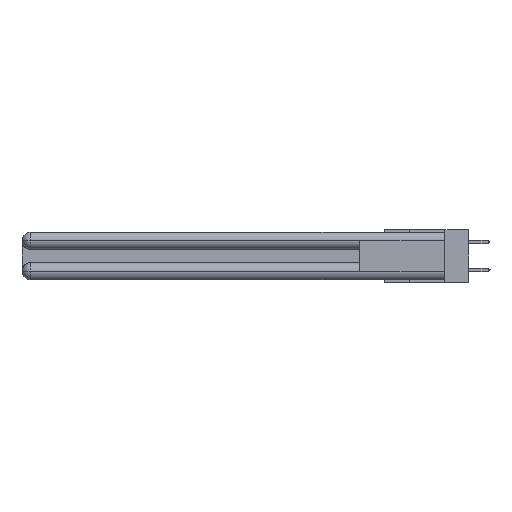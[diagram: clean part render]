
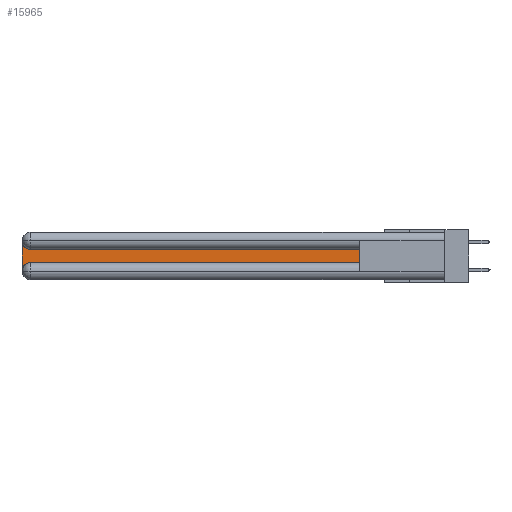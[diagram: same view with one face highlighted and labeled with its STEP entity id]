
A CAD part, left-side view. The second image highlights one B-rep face of the part: STEP entity #15965.
In plain terms, the highlighted planar face has unit normal (-1, 0, 0).
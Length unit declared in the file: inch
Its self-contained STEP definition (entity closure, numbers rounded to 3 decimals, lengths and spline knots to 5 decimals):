
#77 = CARTESIAN_POINT ( 'NONE',  ( 0.075, 2.94, -0.2775 ) ) ;
#426 = DIRECTION ( 'NONE',  ( 0., 1., 0. ) ) ;
#464 = VECTOR ( 'NONE', #27514, 39.37008 ) ;
#1423 = VERTEX_POINT ( 'NONE', #12415 ) ;
#1470 = CARTESIAN_POINT ( 'NONE',  ( 0.075, 2.94, -0.0625 ) ) ;
#2948 = DIRECTION ( 'NONE',  ( 1., 0., 0. ) ) ;
#3179 = VERTEX_POINT ( 'NONE', #11941 ) ;
#4895 = EDGE_CURVE ( 'NONE', #31831, #22219, #6930, .T. ) ;
#5091 = AXIS2_PLACEMENT_3D ( 'NONE', #23180, #6838, #25921 ) ;
#5774 = CARTESIAN_POINT ( 'NONE',  ( 0.075, 2.94, -0.2175 ) ) ;
#5878 = EDGE_LOOP ( 'NONE', ( #30860, #29980, #32222, #12276, #18304, #21427 ) ) ;
#6700 = CIRCLE ( 'NONE', #10263, 0.06 ) ;
#6823 = EDGE_CURVE ( 'NONE', #3179, #1423, #23048, .T. ) ;
#6838 = DIRECTION ( 'NONE',  ( 1., 0., 0. ) ) ;
#6930 = LINE ( 'NONE', #20446, #12074 ) ;
#7459 = VERTEX_POINT ( 'NONE', #5774 ) ;
#8381 = DIRECTION ( 'NONE',  ( 0., -1., 0. ) ) ;
#10263 = AXIS2_PLACEMENT_3D ( 'NONE', #1470, #34293, #17592 ) ;
#11073 = EDGE_CURVE ( 'NONE', #7459, #14673, #18870, .T. ) ;
#11163 = CARTESIAN_POINT ( 'NONE',  ( 0.075, 3., -0.0625 ) ) ;
#11398 = EDGE_CURVE ( 'NONE', #14673, #3179, #31233, .T. ) ;
#11407 = EDGE_CURVE ( 'NONE', #22219, #7459, #28632, .T. ) ;
#11941 = CARTESIAN_POINT ( 'NONE',  ( 0.075, 0.6, -0.1225 ) ) ;
#11987 = CARTESIAN_POINT ( 'NONE',  ( 0.075, 0.6, -0.2175 ) ) ;
#12074 = VECTOR ( 'NONE', #31666, 39.37008 ) ;
#12076 = VECTOR ( 'NONE', #8381, 39.37008 ) ;
#12276 = ORIENTED_EDGE ( 'NONE', *, *, #11407, .T. ) ;
#12415 = CARTESIAN_POINT ( 'NONE',  ( 0.075, 2.94, -0.1225 ) ) ;
#14673 = VERTEX_POINT ( 'NONE', #11987 ) ;
#15965 = ADVANCED_FACE ( 'NONE', ( #21910 ), #17691, .F. ) ;
#16679 = VECTOR ( 'NONE', #426, 39.37008 ) ;
#17262 = CARTESIAN_POINT ( 'NONE',  ( 0.075, 0.6, -0.1225 ) ) ;
#17592 = DIRECTION ( 'NONE',  ( 0., 0., -1. ) ) ;
#17691 = PLANE ( 'NONE',  #5091 ) ;
#18304 = ORIENTED_EDGE ( 'NONE', *, *, #11073, .T. ) ;
#18870 = LINE ( 'NONE', #24700, #12076 ) ;
#20172 = DIRECTION ( 'NONE',  ( 0., 0., -1. ) ) ;
#20200 = EDGE_CURVE ( 'NONE', #1423, #31831, #6700, .T. ) ;
#20446 = CARTESIAN_POINT ( 'NONE',  ( 0.075, 3., -0.2175 ) ) ;
#21427 = ORIENTED_EDGE ( 'NONE', *, *, #11398, .T. ) ;
#21910 = FACE_OUTER_BOUND ( 'NONE', #5878, .T. ) ;
#22219 = VERTEX_POINT ( 'NONE', #29022 ) ;
#23048 = LINE ( 'NONE', #17262, #16679 ) ;
#23180 = CARTESIAN_POINT ( 'NONE',  ( 0.075, 3., -0.1225 ) ) ;
#24700 = CARTESIAN_POINT ( 'NONE',  ( 0.075, 0.6, -0.2175 ) ) ;
#25921 = DIRECTION ( 'NONE',  ( 0., 0., -1. ) ) ;
#27514 = DIRECTION ( 'NONE',  ( 0., 0., 1. ) ) ;
#28632 = CIRCLE ( 'NONE', #29715, 0.06 ) ;
#29022 = CARTESIAN_POINT ( 'NONE',  ( 0.075, 3., -0.2775 ) ) ;
#29715 = AXIS2_PLACEMENT_3D ( 'NONE', #77, #2948, #20172 ) ;
#29980 = ORIENTED_EDGE ( 'NONE', *, *, #20200, .T. ) ;
#30860 = ORIENTED_EDGE ( 'NONE', *, *, #6823, .T. ) ;
#31233 = LINE ( 'NONE', #32655, #464 ) ;
#31666 = DIRECTION ( 'NONE',  ( 0., 0., -1. ) ) ;
#31831 = VERTEX_POINT ( 'NONE', #11163 ) ;
#32222 = ORIENTED_EDGE ( 'NONE', *, *, #4895, .T. ) ;
#32655 = CARTESIAN_POINT ( 'NONE',  ( 0.075, 0.6, -0.2175 ) ) ;
#34293 = DIRECTION ( 'NONE',  ( 1., 0., 0. ) ) ;
